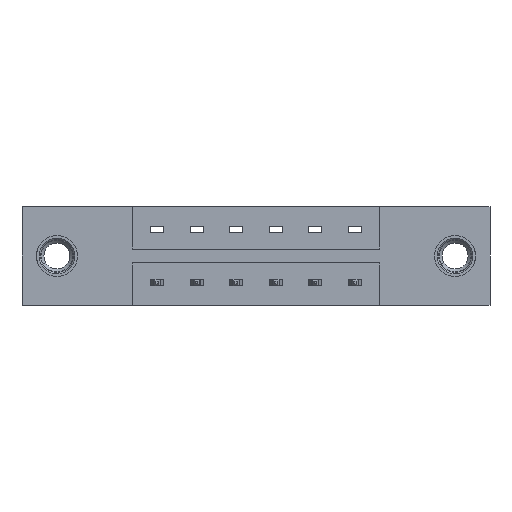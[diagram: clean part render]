
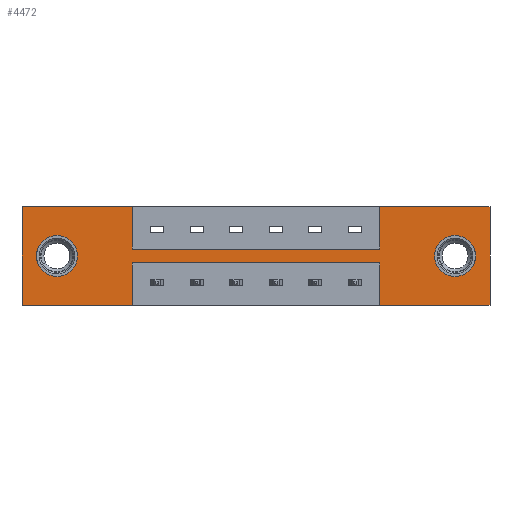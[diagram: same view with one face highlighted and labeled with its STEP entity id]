
A CAD part, front view. The second image highlights one B-rep face of the part: STEP entity #4472.
In plain terms, the highlighted planar face has unit normal (0, -1, 0).
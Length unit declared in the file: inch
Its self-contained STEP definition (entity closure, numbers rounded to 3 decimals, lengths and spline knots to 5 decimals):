
#8 = CARTESIAN_POINT ( 'NONE',  ( 1.3575, 0., 0. ) ) ;
#62 = VERTEX_POINT ( 'NONE', #4469 ) ;
#68 = CARTESIAN_POINT ( 'NONE',  ( 0., 0., 0. ) ) ;
#373 = ORIENTED_EDGE ( 'NONE', *, *, #425, .F. ) ;
#425 = EDGE_CURVE ( 'NONE', #2718, #6247, #2239, .T. ) ;
#442 = DIRECTION ( 'NONE',  ( 0., 1., 0. ) ) ;
#615 = VECTOR ( 'NONE', #2263, 39.37008 ) ;
#682 = CARTESIAN_POINT ( 'NONE',  ( 0.4175, 0., -0.375 ) ) ;
#694 = DIRECTION ( 'NONE',  ( 0., 1., 0. ) ) ;
#812 = DIRECTION ( 'NONE',  ( -1., 0., 0. ) ) ;
#825 = CARTESIAN_POINT ( 'NONE',  ( 1.3575, 0., -0.161 ) ) ;
#1164 = CARTESIAN_POINT ( 'NONE',  ( 0., 0., 0. ) ) ;
#1207 = CARTESIAN_POINT ( 'NONE',  ( 0.4175, 0., -0.161 ) ) ;
#1256 = LINE ( 'NONE', #9166, #1352 ) ;
#1322 = VECTOR ( 'NONE', #4663, 39.37008 ) ;
#1352 = VECTOR ( 'NONE', #4651, 39.37008 ) ;
#1354 = VECTOR ( 'NONE', #812, 39.37008 ) ;
#1516 = CARTESIAN_POINT ( 'NONE',  ( 1.6425, 0., -0.1875 ) ) ;
#1570 = DIRECTION ( 'NONE',  ( 0., 0., 1. ) ) ;
#1635 = PLANE ( 'NONE',  #5465 ) ;
#1734 = CIRCLE ( 'NONE', #6937, 0.078 ) ;
#1810 = EDGE_CURVE ( 'NONE', #2456, #3172, #6991, .T. ) ;
#1971 = EDGE_CURVE ( 'NONE', #3172, #2718, #7586, .T. ) ;
#2016 = LINE ( 'NONE', #1164, #4552 ) ;
#2095 = EDGE_LOOP ( 'NONE', ( #373, #4957, #6111, #4082, #2258, #6637, #9261, #3139, #3640, #3463, #8354, #2688 ) ) ;
#2239 = LINE ( 'NONE', #9084, #1322 ) ;
#2258 = ORIENTED_EDGE ( 'NONE', *, *, #7535, .F. ) ;
#2263 = DIRECTION ( 'NONE',  ( 1., 0., 0. ) ) ;
#2387 = VERTEX_POINT ( 'NONE', #2531 ) ;
#2456 = VERTEX_POINT ( 'NONE', #8270 ) ;
#2470 = CIRCLE ( 'NONE', #4809, 0.078 ) ;
#2531 = CARTESIAN_POINT ( 'NONE',  ( 1.3575, 0., -0.161 ) ) ;
#2583 = CARTESIAN_POINT ( 'NONE',  ( 0.4175, 0., -0.161 ) ) ;
#2590 = EDGE_CURVE ( 'NONE', #6901, #8703, #2016, .T. ) ;
#2635 = DIRECTION ( 'NONE',  ( 0., 1., 0. ) ) ;
#2640 = CARTESIAN_POINT ( 'NONE',  ( 0., 0., -0.375 ) ) ;
#2688 = ORIENTED_EDGE ( 'NONE', *, *, #6362, .F. ) ;
#2715 = VECTOR ( 'NONE', #1570, 39.37008 ) ;
#2718 = VERTEX_POINT ( 'NONE', #7192 ) ;
#2815 = DIRECTION ( 'NONE',  ( 0., 0., 1. ) ) ;
#2959 = EDGE_CURVE ( 'NONE', #7139, #2456, #8470, .T. ) ;
#3080 = CARTESIAN_POINT ( 'NONE',  ( 0.4175, 0., -0.214 ) ) ;
#3130 = VERTEX_POINT ( 'NONE', #5451 ) ;
#3139 = ORIENTED_EDGE ( 'NONE', *, *, #5927, .F. ) ;
#3172 = VERTEX_POINT ( 'NONE', #6161 ) ;
#3355 = DIRECTION ( 'NONE',  ( 0., 0., -1. ) ) ;
#3373 = CARTESIAN_POINT ( 'NONE',  ( 1.6425, 0., -0.1875 ) ) ;
#3463 = ORIENTED_EDGE ( 'NONE', *, *, #4570, .F. ) ;
#3469 = VERTEX_POINT ( 'NONE', #9551 ) ;
#3470 = EDGE_CURVE ( 'NONE', #5962, #62, #2470, .T. ) ;
#3527 = ORIENTED_EDGE ( 'NONE', *, *, #8406, .T. ) ;
#3635 = VERTEX_POINT ( 'NONE', #3080 ) ;
#3640 = ORIENTED_EDGE ( 'NONE', *, *, #2590, .F. ) ;
#3717 = EDGE_CURVE ( 'NONE', #62, #5962, #6036, .T. ) ;
#3869 = CARTESIAN_POINT ( 'NONE',  ( 1.6425, 0., -0.1095 ) ) ;
#4050 = DIRECTION ( 'NONE',  ( 1., 0., 0. ) ) ;
#4082 = ORIENTED_EDGE ( 'NONE', *, *, #2959, .F. ) ;
#4283 = CARTESIAN_POINT ( 'NONE',  ( 0.1325, 0., -0.1875 ) ) ;
#4322 = VERTEX_POINT ( 'NONE', #8049 ) ;
#4469 = CARTESIAN_POINT ( 'NONE',  ( 1.6425, 0., -0.2655 ) ) ;
#4472 = ADVANCED_FACE ( 'NONE', ( #5834, #7698, #4918 ), #1635, .T. ) ;
#4552 = VECTOR ( 'NONE', #6357, 39.37008 ) ;
#4570 = EDGE_CURVE ( 'NONE', #5342, #6901, #1256, .T. ) ;
#4588 = LINE ( 'NONE', #5339, #5528 ) ;
#4651 = DIRECTION ( 'NONE',  ( -1., 0., 0. ) ) ;
#4663 = DIRECTION ( 'NONE',  ( 0., 0., 1. ) ) ;
#4807 = EDGE_CURVE ( 'NONE', #5907, #3130, #8529, .T. ) ;
#4809 = AXIS2_PLACEMENT_3D ( 'NONE', #1516, #694, #6557 ) ;
#4853 = ORIENTED_EDGE ( 'NONE', *, *, #3470, .T. ) ;
#4857 = CARTESIAN_POINT ( 'NONE',  ( 0.1325, 0., -0.1875 ) ) ;
#4870 = EDGE_CURVE ( 'NONE', #3469, #4322, #1734, .T. ) ;
#4918 = FACE_OUTER_BOUND ( 'NONE', #2095, .T. ) ;
#4957 = ORIENTED_EDGE ( 'NONE', *, *, #1971, .F. ) ;
#5022 = VECTOR ( 'NONE', #9426, 39.37008 ) ;
#5125 = LINE ( 'NONE', #2583, #9290 ) ;
#5339 = CARTESIAN_POINT ( 'NONE',  ( 0., 0., 0. ) ) ;
#5342 = VERTEX_POINT ( 'NONE', #682 ) ;
#5368 = CARTESIAN_POINT ( 'NONE',  ( 0., 0., -0.375 ) ) ;
#5370 = EDGE_LOOP ( 'NONE', ( #4853, #7962 ) ) ;
#5451 = CARTESIAN_POINT ( 'NONE',  ( 0.4175, 0., -0.161 ) ) ;
#5465 = AXIS2_PLACEMENT_3D ( 'NONE', #5368, #6761, #6722 ) ;
#5528 = VECTOR ( 'NONE', #6115, 39.37008 ) ;
#5834 = FACE_BOUND ( 'NONE', #5370, .T. ) ;
#5907 = VERTEX_POINT ( 'NONE', #6669 ) ;
#5920 = CARTESIAN_POINT ( 'NONE',  ( 0., 0., -0.375 ) ) ;
#5927 = EDGE_CURVE ( 'NONE', #8703, #5907, #4588, .T. ) ;
#5962 = VERTEX_POINT ( 'NONE', #3869 ) ;
#6036 = CIRCLE ( 'NONE', #8355, 0.078 ) ;
#6111 = ORIENTED_EDGE ( 'NONE', *, *, #1810, .F. ) ;
#6115 = DIRECTION ( 'NONE',  ( 1., 0., 0. ) ) ;
#6161 = CARTESIAN_POINT ( 'NONE',  ( 1.775, 0., -0.375 ) ) ;
#6181 = VECTOR ( 'NONE', #3355, 39.37008 ) ;
#6247 = VERTEX_POINT ( 'NONE', #7164 ) ;
#6258 = CARTESIAN_POINT ( 'NONE',  ( 0.4175, 0., -0.214 ) ) ;
#6344 = DIRECTION ( 'NONE',  ( 0., 0., 1. ) ) ;
#6357 = DIRECTION ( 'NONE',  ( 0., 0., 1. ) ) ;
#6362 = EDGE_CURVE ( 'NONE', #6247, #3635, #8168, .T. ) ;
#6557 = DIRECTION ( 'NONE',  ( 0., 0., -1. ) ) ;
#6637 = ORIENTED_EDGE ( 'NONE', *, *, #7850, .F. ) ;
#6669 = CARTESIAN_POINT ( 'NONE',  ( 0.4175, 0., 0. ) ) ;
#6722 = DIRECTION ( 'NONE',  ( 0., 0., -1. ) ) ;
#6761 = DIRECTION ( 'NONE',  ( 0., -1., 0. ) ) ;
#6853 = CIRCLE ( 'NONE', #9478, 0.078 ) ;
#6901 = VERTEX_POINT ( 'NONE', #2640 ) ;
#6937 = AXIS2_PLACEMENT_3D ( 'NONE', #4283, #7204, #2815 ) ;
#6991 = LINE ( 'NONE', #8752, #5022 ) ;
#7050 = DIRECTION ( 'NONE',  ( 0., 0., -1. ) ) ;
#7139 = VERTEX_POINT ( 'NONE', #8 ) ;
#7164 = CARTESIAN_POINT ( 'NONE',  ( 1.3575, 0., -0.214 ) ) ;
#7192 = CARTESIAN_POINT ( 'NONE',  ( 1.3575, 0., -0.375 ) ) ;
#7204 = DIRECTION ( 'NONE',  ( 0., 1., 0. ) ) ;
#7327 = LINE ( 'NONE', #6258, #6181 ) ;
#7535 = EDGE_CURVE ( 'NONE', #2387, #7139, #8142, .T. ) ;
#7586 = LINE ( 'NONE', #5920, #1354 ) ;
#7698 = FACE_BOUND ( 'NONE', #7790, .T. ) ;
#7790 = EDGE_LOOP ( 'NONE', ( #3527, #8607 ) ) ;
#7844 = VECTOR ( 'NONE', #7050, 39.37008 ) ;
#7850 = EDGE_CURVE ( 'NONE', #3130, #2387, #5125, .T. ) ;
#7864 = EDGE_CURVE ( 'NONE', #3635, #5342, #7327, .T. ) ;
#7962 = ORIENTED_EDGE ( 'NONE', *, *, #3717, .T. ) ;
#8049 = CARTESIAN_POINT ( 'NONE',  ( 0.1325, 0., -0.1095 ) ) ;
#8142 = LINE ( 'NONE', #825, #2715 ) ;
#8151 = CARTESIAN_POINT ( 'NONE',  ( 0., 0., 0. ) ) ;
#8168 = LINE ( 'NONE', #8764, #8506 ) ;
#8270 = CARTESIAN_POINT ( 'NONE',  ( 1.775, 0., 0. ) ) ;
#8354 = ORIENTED_EDGE ( 'NONE', *, *, #7864, .F. ) ;
#8355 = AXIS2_PLACEMENT_3D ( 'NONE', #3373, #2635, #8587 ) ;
#8406 = EDGE_CURVE ( 'NONE', #4322, #3469, #6853, .T. ) ;
#8470 = LINE ( 'NONE', #68, #615 ) ;
#8506 = VECTOR ( 'NONE', #8844, 39.37008 ) ;
#8529 = LINE ( 'NONE', #1207, #7844 ) ;
#8587 = DIRECTION ( 'NONE',  ( 0., 0., -1. ) ) ;
#8607 = ORIENTED_EDGE ( 'NONE', *, *, #4870, .T. ) ;
#8703 = VERTEX_POINT ( 'NONE', #8151 ) ;
#8752 = CARTESIAN_POINT ( 'NONE',  ( 1.775, 0., 0. ) ) ;
#8764 = CARTESIAN_POINT ( 'NONE',  ( 0.4175, 0., -0.214 ) ) ;
#8844 = DIRECTION ( 'NONE',  ( -1., 0., 0. ) ) ;
#9084 = CARTESIAN_POINT ( 'NONE',  ( 1.3575, 0., -0.214 ) ) ;
#9166 = CARTESIAN_POINT ( 'NONE',  ( 0., 0., -0.375 ) ) ;
#9261 = ORIENTED_EDGE ( 'NONE', *, *, #4807, .F. ) ;
#9290 = VECTOR ( 'NONE', #4050, 39.37008 ) ;
#9426 = DIRECTION ( 'NONE',  ( 0., 0., -1. ) ) ;
#9478 = AXIS2_PLACEMENT_3D ( 'NONE', #4857, #442, #6344 ) ;
#9551 = CARTESIAN_POINT ( 'NONE',  ( 0.1325, 0., -0.2655 ) ) ;
